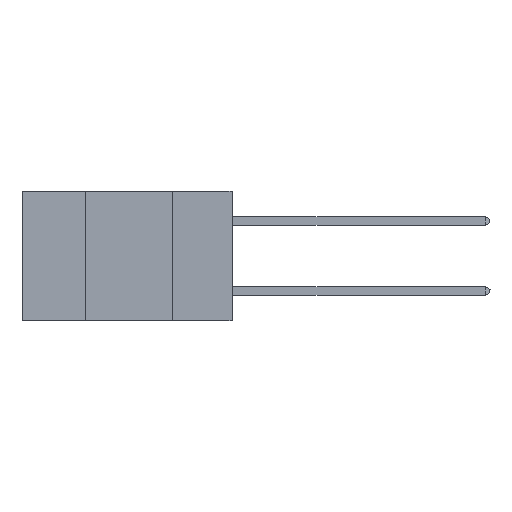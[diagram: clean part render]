
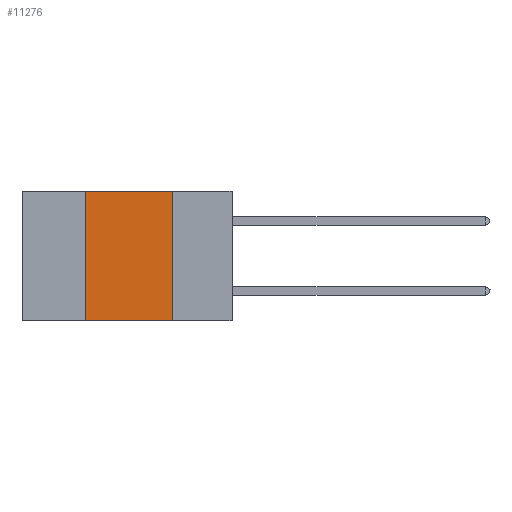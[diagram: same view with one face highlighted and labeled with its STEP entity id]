
A CAD part, left-side view. The second image highlights one B-rep face of the part: STEP entity #11276.
In plain terms, the highlighted planar face has unit normal (-1, 0, 0).
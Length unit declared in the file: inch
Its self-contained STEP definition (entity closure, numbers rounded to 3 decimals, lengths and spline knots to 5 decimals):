
#331 = LINE ( 'NONE', #19759, #10048 ) ;
#882 = ORIENTED_EDGE ( 'NONE', *, *, #1592, .F. ) ;
#1592 = EDGE_CURVE ( 'NONE', #14441, #16070, #331, .T. ) ;
#2426 = DIRECTION ( 'NONE',  ( 1., 0., 0. ) ) ;
#2695 = VECTOR ( 'NONE', #8779, 39.37008 ) ;
#4749 = FACE_OUTER_BOUND ( 'NONE', #7568, .T. ) ;
#5880 = VECTOR ( 'NONE', #20987, 39.37008 ) ;
#7568 = EDGE_LOOP ( 'NONE', ( #882, #11330, #11180, #26875 ) ) ;
#7835 = EDGE_CURVE ( 'NONE', #25844, #11426, #29571, .T. ) ;
#8779 = DIRECTION ( 'NONE',  ( 0., 0., 1. ) ) ;
#10048 = VECTOR ( 'NONE', #25850, 39.37008 ) ;
#11180 = ORIENTED_EDGE ( 'NONE', *, *, #7835, .F. ) ;
#11276 = ADVANCED_FACE ( 'NONE', ( #4749 ), #34909, .F. ) ;
#11330 = ORIENTED_EDGE ( 'NONE', *, *, #37878, .F. ) ;
#11426 = VERTEX_POINT ( 'NONE', #32322 ) ;
#14441 = VERTEX_POINT ( 'NONE', #30779 ) ;
#16070 = VERTEX_POINT ( 'NONE', #30459 ) ;
#19759 = CARTESIAN_POINT ( 'NONE',  ( 0., 0.17, 0. ) ) ;
#19957 = CARTESIAN_POINT ( 'NONE',  ( 0., 0.42, -0.37 ) ) ;
#20189 = CARTESIAN_POINT ( 'NONE',  ( 0., 0.6, 0. ) ) ;
#20987 = DIRECTION ( 'NONE',  ( 0., -1., 0. ) ) ;
#22219 = CARTESIAN_POINT ( 'NONE',  ( 0., 0.6, -0.37 ) ) ;
#22487 = DIRECTION ( 'NONE',  ( 0., -1., 0. ) ) ;
#23148 = DIRECTION ( 'NONE',  ( 0., 0., -1. ) ) ;
#25844 = VERTEX_POINT ( 'NONE', #19957 ) ;
#25850 = DIRECTION ( 'NONE',  ( 0., 0., -1. ) ) ;
#26875 = ORIENTED_EDGE ( 'NONE', *, *, #38190, .T. ) ;
#29571 = LINE ( 'NONE', #32355, #2695 ) ;
#30459 = CARTESIAN_POINT ( 'NONE',  ( 0., 0.17, -0.37 ) ) ;
#30779 = CARTESIAN_POINT ( 'NONE',  ( 0., 0.17, 0. ) ) ;
#31799 = VECTOR ( 'NONE', #22487, 39.37008 ) ;
#32322 = CARTESIAN_POINT ( 'NONE',  ( 0., 0.42, 0. ) ) ;
#32355 = CARTESIAN_POINT ( 'NONE',  ( 0., 0.42, 0. ) ) ;
#33210 = LINE ( 'NONE', #35949, #5880 ) ;
#34641 = AXIS2_PLACEMENT_3D ( 'NONE', #20189, #2426, #23148 ) ;
#34909 = PLANE ( 'NONE',  #34641 ) ;
#35043 = LINE ( 'NONE', #22219, #31799 ) ;
#35949 = CARTESIAN_POINT ( 'NONE',  ( 0., 0.6, 0. ) ) ;
#37878 = EDGE_CURVE ( 'NONE', #11426, #14441, #33210, .T. ) ;
#38190 = EDGE_CURVE ( 'NONE', #25844, #16070, #35043, .T. ) ;
